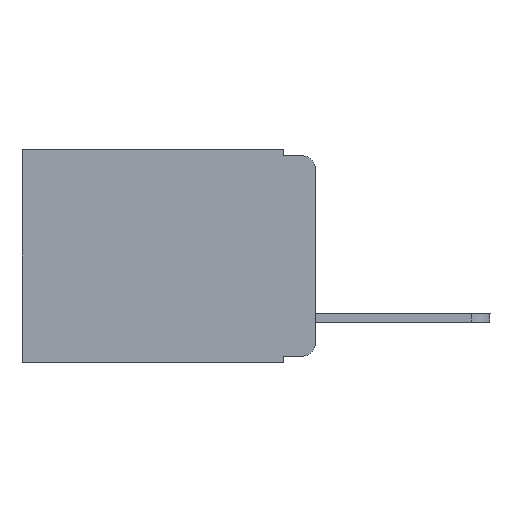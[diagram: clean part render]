
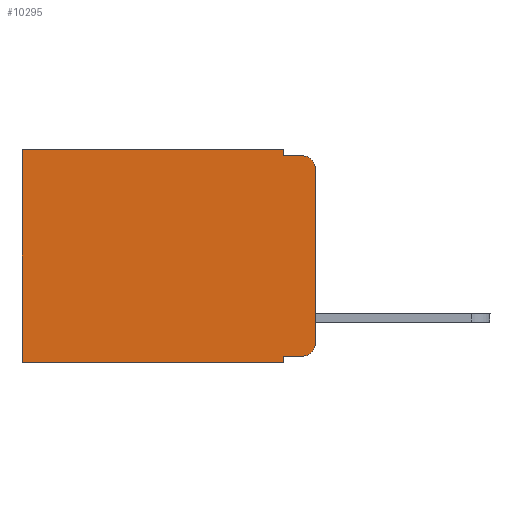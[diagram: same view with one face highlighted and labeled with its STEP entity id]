
A CAD part, left-side view. The second image highlights one B-rep face of the part: STEP entity #10295.
In plain terms, the highlighted planar face has unit normal (-1, 0, 0).
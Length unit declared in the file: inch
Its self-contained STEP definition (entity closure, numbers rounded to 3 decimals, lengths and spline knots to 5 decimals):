
#31 = CARTESIAN_POINT ( 'NONE',  ( 0.298, 0.473, -0.343 ) ) ;
#198 = CARTESIAN_POINT ( 'NONE',  ( 0.298, 0., 0. ) ) ;
#248 = CARTESIAN_POINT ( 'NONE',  ( 0.298, 0., -0.313 ) ) ;
#301 = VERTEX_POINT ( 'NONE', #17162 ) ;
#383 = LINE ( 'NONE', #198, #10659 ) ;
#716 = CARTESIAN_POINT ( 'NONE',  ( 0.298, 0.02, -0.01 ) ) ;
#1002 = VERTEX_POINT ( 'NONE', #17444 ) ;
#1025 = VERTEX_POINT ( 'NONE', #31 ) ;
#1186 = CARTESIAN_POINT ( 'NONE',  ( 0.298, 0.02, -0.313 ) ) ;
#1211 = PLANE ( 'NONE',  #8141 ) ;
#1445 = EDGE_LOOP ( 'NONE', ( #11161, #17751, #5157, #16834, #5602, #11221, #17219, #9593, #13547, #10094 ) ) ;
#1784 = DIRECTION ( 'NONE',  ( 0., 0., -1. ) ) ;
#1926 = VECTOR ( 'NONE', #16031, 39.37008 ) ;
#2064 = VERTEX_POINT ( 'NONE', #248 ) ;
#2094 = CARTESIAN_POINT ( 'NONE',  ( 0.298, 0.051, 0. ) ) ;
#2205 = LINE ( 'NONE', #8276, #11720 ) ;
#2514 = CARTESIAN_POINT ( 'NONE',  ( 0.298, 0.051, 0. ) ) ;
#2783 = CARTESIAN_POINT ( 'NONE',  ( 0.298, 0.473, 0. ) ) ;
#2827 = CARTESIAN_POINT ( 'NONE',  ( 0.298, 0.051, -0.333 ) ) ;
#2937 = FACE_OUTER_BOUND ( 'NONE', #1445, .T. ) ;
#3355 = VECTOR ( 'NONE', #5380, 39.37008 ) ;
#3389 = LINE ( 'NONE', #11931, #17564 ) ;
#3613 = DIRECTION ( 'NONE',  ( 0., 0., -1. ) ) ;
#3667 = EDGE_CURVE ( 'NONE', #5935, #301, #15942, .T. ) ;
#3771 = CARTESIAN_POINT ( 'NONE',  ( 0.298, 0., -0.343 ) ) ;
#4141 = EDGE_CURVE ( 'NONE', #15126, #9100, #7163, .T. ) ;
#4219 = CARTESIAN_POINT ( 'NONE',  ( 0.298, 0.051, -0.01 ) ) ;
#4901 = VECTOR ( 'NONE', #3613, 39.37008 ) ;
#5157 = ORIENTED_EDGE ( 'NONE', *, *, #4141, .F. ) ;
#5380 = DIRECTION ( 'NONE',  ( 0., 1., 0. ) ) ;
#5602 = ORIENTED_EDGE ( 'NONE', *, *, #15837, .T. ) ;
#5935 = VERTEX_POINT ( 'NONE', #17106 ) ;
#5938 = VECTOR ( 'NONE', #15819, 39.37008 ) ;
#6757 = EDGE_CURVE ( 'NONE', #5935, #11889, #3389, .T. ) ;
#7163 = LINE ( 'NONE', #4219, #5938 ) ;
#7184 = CARTESIAN_POINT ( 'NONE',  ( 0.298, 0.473, 0. ) ) ;
#7644 = DIRECTION ( 'NONE',  ( 0., 0., -1. ) ) ;
#7962 = LINE ( 'NONE', #3771, #3355 ) ;
#8141 = AXIS2_PLACEMENT_3D ( 'NONE', #12809, #10446, #1784 ) ;
#8180 = VECTOR ( 'NONE', #18491, 39.37008 ) ;
#8276 = CARTESIAN_POINT ( 'NONE',  ( 0.298, 0., 0. ) ) ;
#8657 = VERTEX_POINT ( 'NONE', #2783 ) ;
#8845 = EDGE_CURVE ( 'NONE', #1002, #2064, #2205, .T. ) ;
#9100 = VERTEX_POINT ( 'NONE', #716 ) ;
#9249 = DIRECTION ( 'NONE',  ( 0., 0., -1. ) ) ;
#9540 = EDGE_CURVE ( 'NONE', #1002, #9100, #13635, .T. ) ;
#9563 = CARTESIAN_POINT ( 'NONE',  ( 0.298, 0.051, -0.01 ) ) ;
#9593 = ORIENTED_EDGE ( 'NONE', *, *, #6757, .F. ) ;
#10094 = ORIENTED_EDGE ( 'NONE', *, *, #13876, .T. ) ;
#10295 = ADVANCED_FACE ( 'NONE', ( #2937 ), #1211, .F. ) ;
#10446 = DIRECTION ( 'NONE',  ( 1., 0., 0. ) ) ;
#10659 = VECTOR ( 'NONE', #16371, 39.37008 ) ;
#10662 = EDGE_CURVE ( 'NONE', #8657, #1025, #12975, .T. ) ;
#11161 = ORIENTED_EDGE ( 'NONE', *, *, #8845, .F. ) ;
#11221 = ORIENTED_EDGE ( 'NONE', *, *, #10662, .T. ) ;
#11720 = VECTOR ( 'NONE', #12162, 39.37008 ) ;
#11850 = EDGE_CURVE ( 'NONE', #15678, #15126, #15019, .T. ) ;
#11889 = VERTEX_POINT ( 'NONE', #16544 ) ;
#11931 = CARTESIAN_POINT ( 'NONE',  ( 0.298, 0.051, 0. ) ) ;
#12162 = DIRECTION ( 'NONE',  ( 0., 0., -1. ) ) ;
#12407 = CIRCLE ( 'NONE', #17013, 0.02 ) ;
#12809 = CARTESIAN_POINT ( 'NONE',  ( 0.298, 0., 0. ) ) ;
#12975 = LINE ( 'NONE', #7184, #8180 ) ;
#13547 = ORIENTED_EDGE ( 'NONE', *, *, #3667, .T. ) ;
#13635 = CIRCLE ( 'NONE', #18477, 0.02 ) ;
#13876 = EDGE_CURVE ( 'NONE', #301, #2064, #12407, .T. ) ;
#15019 = LINE ( 'NONE', #2094, #4901 ) ;
#15042 = EDGE_CURVE ( 'NONE', #11889, #1025, #7962, .T. ) ;
#15126 = VERTEX_POINT ( 'NONE', #9563 ) ;
#15678 = VERTEX_POINT ( 'NONE', #2514 ) ;
#15819 = DIRECTION ( 'NONE',  ( 0., -1., 0. ) ) ;
#15837 = EDGE_CURVE ( 'NONE', #15678, #8657, #383, .T. ) ;
#15942 = LINE ( 'NONE', #2827, #1926 ) ;
#16031 = DIRECTION ( 'NONE',  ( 0., -1., 0. ) ) ;
#16371 = DIRECTION ( 'NONE',  ( 0., 1., 0. ) ) ;
#16479 = DIRECTION ( 'NONE',  ( -1., 0., 0. ) ) ;
#16544 = CARTESIAN_POINT ( 'NONE',  ( 0.298, 0.051, -0.343 ) ) ;
#16834 = ORIENTED_EDGE ( 'NONE', *, *, #11850, .F. ) ;
#17013 = AXIS2_PLACEMENT_3D ( 'NONE', #1186, #18486, #17348 ) ;
#17106 = CARTESIAN_POINT ( 'NONE',  ( 0.298, 0.051, -0.333 ) ) ;
#17162 = CARTESIAN_POINT ( 'NONE',  ( 0.298, 0.02, -0.333 ) ) ;
#17219 = ORIENTED_EDGE ( 'NONE', *, *, #15042, .F. ) ;
#17348 = DIRECTION ( 'NONE',  ( 0., 0., -1. ) ) ;
#17444 = CARTESIAN_POINT ( 'NONE',  ( 0.298, 0., -0.03 ) ) ;
#17564 = VECTOR ( 'NONE', #7644, 39.37008 ) ;
#17751 = ORIENTED_EDGE ( 'NONE', *, *, #9540, .T. ) ;
#17817 = CARTESIAN_POINT ( 'NONE',  ( 0.298, 0.02, -0.03 ) ) ;
#18477 = AXIS2_PLACEMENT_3D ( 'NONE', #17817, #16479, #9249 ) ;
#18486 = DIRECTION ( 'NONE',  ( -1., 0., 0. ) ) ;
#18491 = DIRECTION ( 'NONE',  ( 0., 0., -1. ) ) ;
